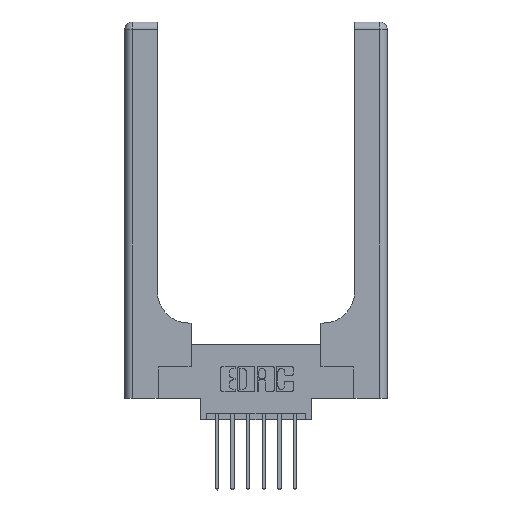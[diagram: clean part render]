
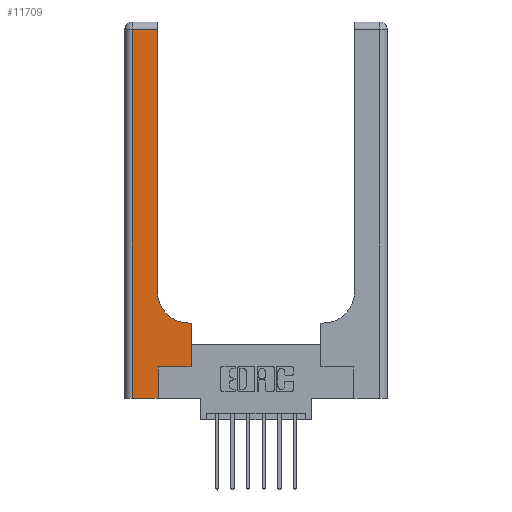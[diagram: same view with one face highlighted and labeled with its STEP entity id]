
A CAD part, top view. The second image highlights one B-rep face of the part: STEP entity #11709.
In plain terms, the highlighted planar face has unit normal (0, 0, 1).
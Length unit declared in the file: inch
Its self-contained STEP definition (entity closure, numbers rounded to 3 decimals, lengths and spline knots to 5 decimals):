
#107 = CARTESIAN_POINT ( 'NONE',  ( 0.51, 0.6, 0.37 ) ) ;
#371 = DIRECTION ( 'NONE',  ( 0., -1., 0. ) ) ;
#667 = LINE ( 'NONE', #5151, #12239 ) ;
#776 = VECTOR ( 'NONE', #6103, 39.37008 ) ;
#1054 = DIRECTION ( 'NONE',  ( 1., 0., 0. ) ) ;
#1102 = VECTOR ( 'NONE', #4640, 39.37008 ) ;
#1354 = CARTESIAN_POINT ( 'NONE',  ( 0.26, 0.85, 0.37 ) ) ;
#1648 = CARTESIAN_POINT ( 'NONE',  ( 0.265, 0.25, 0.37 ) ) ;
#1699 = DIRECTION ( 'NONE',  ( 1., 0., 0. ) ) ;
#1920 = EDGE_CURVE ( 'NONE', #11260, #10404, #7956, .T. ) ;
#2137 = ORIENTED_EDGE ( 'NONE', *, *, #11750, .T. ) ;
#2186 = EDGE_CURVE ( 'NONE', #7191, #11516, #3716, .T. ) ;
#2257 = VERTEX_POINT ( 'NONE', #13802 ) ;
#2932 = FACE_OUTER_BOUND ( 'NONE', #4375, .T. ) ;
#3111 = ORIENTED_EDGE ( 'NONE', *, *, #2186, .T. ) ;
#3178 = DIRECTION ( 'NONE',  ( 0., 0., -1. ) ) ;
#3327 = CARTESIAN_POINT ( 'NONE',  ( 0.26, 0.6, 0.37 ) ) ;
#3530 = CARTESIAN_POINT ( 'NONE',  ( 0.528, 0.25, 0.37 ) ) ;
#3581 = ORIENTED_EDGE ( 'NONE', *, *, #6320, .T. ) ;
#3716 = LINE ( 'NONE', #7201, #776 ) ;
#4291 = VERTEX_POINT ( 'NONE', #1354 ) ;
#4375 = EDGE_LOOP ( 'NONE', ( #3581, #3111, #12432, #11578, #13310, #10628, #13143, #11159, #2137 ) ) ;
#4427 = EDGE_CURVE ( 'NONE', #13974, #8448, #667, .T. ) ;
#4499 = AXIS2_PLACEMENT_3D ( 'NONE', #14074, #7609, #1054 ) ;
#4640 = DIRECTION ( 'NONE',  ( 0., 1., 0. ) ) ;
#4712 = CARTESIAN_POINT ( 'NONE',  ( 0.265, 0., 0.37 ) ) ;
#4789 = VECTOR ( 'NONE', #1699, 39.37008 ) ;
#5151 = CARTESIAN_POINT ( 'NONE',  ( 0.265, 0., 0.37 ) ) ;
#5166 = CIRCLE ( 'NONE', #4499, 0.25 ) ;
#5248 = AXIS2_PLACEMENT_3D ( 'NONE', #13989, #3178, #10772 ) ;
#5266 = VECTOR ( 'NONE', #8843, 39.37008 ) ;
#5360 = VERTEX_POINT ( 'NONE', #107 ) ;
#5608 = LINE ( 'NONE', #6365, #11685 ) ;
#5849 = CARTESIAN_POINT ( 'NONE',  ( 0.06, 3., 0.37 ) ) ;
#6103 = DIRECTION ( 'NONE',  ( -1., 0., 0. ) ) ;
#6320 = EDGE_CURVE ( 'NONE', #4291, #7191, #5608, .T. ) ;
#6365 = CARTESIAN_POINT ( 'NONE',  ( 0.26, 3., 0.37 ) ) ;
#6463 = LINE ( 'NONE', #3327, #12185 ) ;
#6508 = EDGE_CURVE ( 'NONE', #10404, #5360, #6463, .T. ) ;
#6666 = CARTESIAN_POINT ( 'NONE',  ( 0., 0., 0.37 ) ) ;
#7191 = VERTEX_POINT ( 'NONE', #8048 ) ;
#7201 = CARTESIAN_POINT ( 'NONE',  ( 0., 2.94, 0.37 ) ) ;
#7333 = LINE ( 'NONE', #5849, #9851 ) ;
#7575 = EDGE_CURVE ( 'NONE', #2257, #13974, #8498, .T. ) ;
#7609 = DIRECTION ( 'NONE',  ( 0., 0., -1. ) ) ;
#7956 = LINE ( 'NONE', #3530, #1102 ) ;
#8048 = CARTESIAN_POINT ( 'NONE',  ( 0.26, 2.94, 0.37 ) ) ;
#8224 = CARTESIAN_POINT ( 'NONE',  ( 0.528, 0.6, 0.37 ) ) ;
#8448 = VERTEX_POINT ( 'NONE', #1648 ) ;
#8498 = LINE ( 'NONE', #6666, #5266 ) ;
#8776 = DIRECTION ( 'NONE',  ( -1., 0., 0. ) ) ;
#8843 = DIRECTION ( 'NONE',  ( 1., 0., 0. ) ) ;
#9323 = CARTESIAN_POINT ( 'NONE',  ( 0.265, 0.25, 0.37 ) ) ;
#9851 = VECTOR ( 'NONE', #371, 39.37008 ) ;
#10202 = LINE ( 'NONE', #9323, #4789 ) ;
#10404 = VERTEX_POINT ( 'NONE', #8224 ) ;
#10628 = ORIENTED_EDGE ( 'NONE', *, *, #13488, .T. ) ;
#10733 = PLANE ( 'NONE',  #5248 ) ;
#10772 = DIRECTION ( 'NONE',  ( -1., 0., 0. ) ) ;
#11159 = ORIENTED_EDGE ( 'NONE', *, *, #6508, .T. ) ;
#11260 = VERTEX_POINT ( 'NONE', #12053 ) ;
#11516 = VERTEX_POINT ( 'NONE', #12575 ) ;
#11578 = ORIENTED_EDGE ( 'NONE', *, *, #7575, .T. ) ;
#11685 = VECTOR ( 'NONE', #12823, 39.37008 ) ;
#11709 = ADVANCED_FACE ( 'NONE', ( #2932 ), #10733, .F. ) ;
#11750 = EDGE_CURVE ( 'NONE', #5360, #4291, #5166, .T. ) ;
#12053 = CARTESIAN_POINT ( 'NONE',  ( 0.528, 0.25, 0.37 ) ) ;
#12185 = VECTOR ( 'NONE', #8776, 39.37008 ) ;
#12239 = VECTOR ( 'NONE', #12708, 39.37008 ) ;
#12432 = ORIENTED_EDGE ( 'NONE', *, *, #14015, .T. ) ;
#12575 = CARTESIAN_POINT ( 'NONE',  ( 0.06, 2.94, 0.37 ) ) ;
#12708 = DIRECTION ( 'NONE',  ( 0., 1., 0. ) ) ;
#12823 = DIRECTION ( 'NONE',  ( 0., 1., 0. ) ) ;
#13143 = ORIENTED_EDGE ( 'NONE', *, *, #1920, .T. ) ;
#13310 = ORIENTED_EDGE ( 'NONE', *, *, #4427, .T. ) ;
#13488 = EDGE_CURVE ( 'NONE', #8448, #11260, #10202, .T. ) ;
#13802 = CARTESIAN_POINT ( 'NONE',  ( 0.06, 0., 0.37 ) ) ;
#13974 = VERTEX_POINT ( 'NONE', #4712 ) ;
#13989 = CARTESIAN_POINT ( 'NONE',  ( 0., 3., 0.37 ) ) ;
#14015 = EDGE_CURVE ( 'NONE', #11516, #2257, #7333, .T. ) ;
#14074 = CARTESIAN_POINT ( 'NONE',  ( 0.51, 0.85, 0.37 ) ) ;
